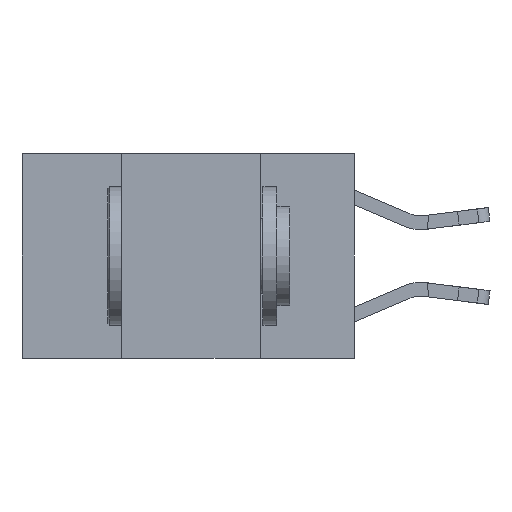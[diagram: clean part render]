
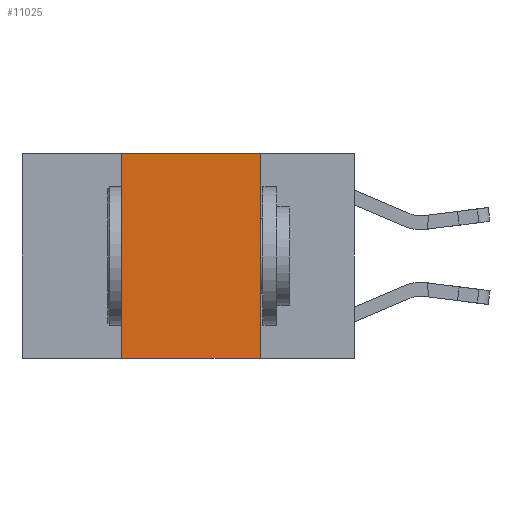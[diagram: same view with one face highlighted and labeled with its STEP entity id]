
A CAD part, left-side view. The second image highlights one B-rep face of the part: STEP entity #11025.
In plain terms, the highlighted planar face has unit normal (-1, 0, 0).
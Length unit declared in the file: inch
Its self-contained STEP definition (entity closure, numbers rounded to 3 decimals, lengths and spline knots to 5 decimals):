
#1276 = VECTOR ( 'NONE', #12708, 39.37008 ) ;
#1372 = DIRECTION ( 'NONE',  ( 0., 0., 1. ) ) ;
#1828 = DIRECTION ( 'NONE',  ( 0., -1., 0. ) ) ;
#1920 = VERTEX_POINT ( 'NONE', #7165 ) ;
#2059 = DIRECTION ( 'NONE',  ( 0., -1., 0. ) ) ;
#2550 = CARTESIAN_POINT ( 'NONE',  ( 0., 0.6, 0. ) ) ;
#2651 = CARTESIAN_POINT ( 'NONE',  ( 0., 0.6, 0. ) ) ;
#2906 = AXIS2_PLACEMENT_3D ( 'NONE', #2550, #3550, #10470 ) ;
#3142 = VERTEX_POINT ( 'NONE', #7270 ) ;
#3383 = EDGE_CURVE ( 'NONE', #3142, #10251, #5433, .T. ) ;
#3550 = DIRECTION ( 'NONE',  ( 1., 0., 0. ) ) ;
#3939 = VERTEX_POINT ( 'NONE', #11709 ) ;
#3983 = CARTESIAN_POINT ( 'NONE',  ( 0., 0.17, 0. ) ) ;
#4186 = FACE_OUTER_BOUND ( 'NONE', #10967, .T. ) ;
#4355 = LINE ( 'NONE', #7356, #11843 ) ;
#4672 = VECTOR ( 'NONE', #2059, 39.37008 ) ;
#5085 = CARTESIAN_POINT ( 'NONE',  ( 0., 0.6, -0.37 ) ) ;
#5129 = VECTOR ( 'NONE', #1828, 39.37008 ) ;
#5433 = LINE ( 'NONE', #2651, #5129 ) ;
#7165 = CARTESIAN_POINT ( 'NONE',  ( 0., 0.17, -0.37 ) ) ;
#7270 = CARTESIAN_POINT ( 'NONE',  ( 0., 0.42, 0. ) ) ;
#7356 = CARTESIAN_POINT ( 'NONE',  ( 0., 0.42, 0. ) ) ;
#7970 = ORIENTED_EDGE ( 'NONE', *, *, #8584, .F. ) ;
#8073 = ORIENTED_EDGE ( 'NONE', *, *, #3383, .F. ) ;
#8134 = ORIENTED_EDGE ( 'NONE', *, *, #10329, .F. ) ;
#8263 = ORIENTED_EDGE ( 'NONE', *, *, #10783, .T. ) ;
#8513 = PLANE ( 'NONE',  #2906 ) ;
#8584 = EDGE_CURVE ( 'NONE', #10251, #1920, #9512, .T. ) ;
#9265 = CARTESIAN_POINT ( 'NONE',  ( 0., 0.17, 0. ) ) ;
#9512 = LINE ( 'NONE', #3983, #1276 ) ;
#9616 = LINE ( 'NONE', #5085, #4672 ) ;
#10251 = VERTEX_POINT ( 'NONE', #9265 ) ;
#10329 = EDGE_CURVE ( 'NONE', #3939, #3142, #4355, .T. ) ;
#10470 = DIRECTION ( 'NONE',  ( 0., 0., -1. ) ) ;
#10783 = EDGE_CURVE ( 'NONE', #3939, #1920, #9616, .T. ) ;
#10967 = EDGE_LOOP ( 'NONE', ( #7970, #8073, #8134, #8263 ) ) ;
#11025 = ADVANCED_FACE ( 'NONE', ( #4186 ), #8513, .F. ) ;
#11709 = CARTESIAN_POINT ( 'NONE',  ( 0., 0.42, -0.37 ) ) ;
#11843 = VECTOR ( 'NONE', #1372, 39.37008 ) ;
#12708 = DIRECTION ( 'NONE',  ( 0., 0., -1. ) ) ;
